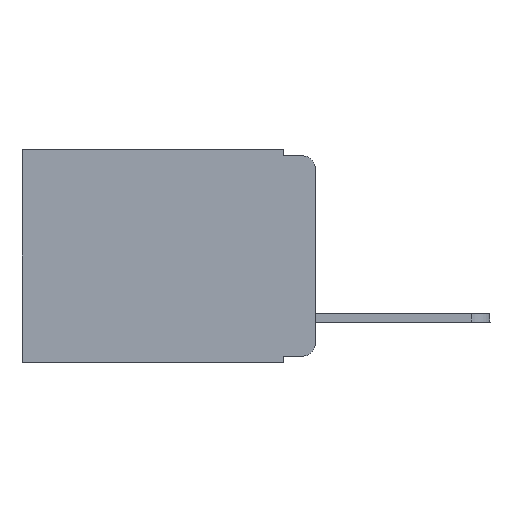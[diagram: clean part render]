
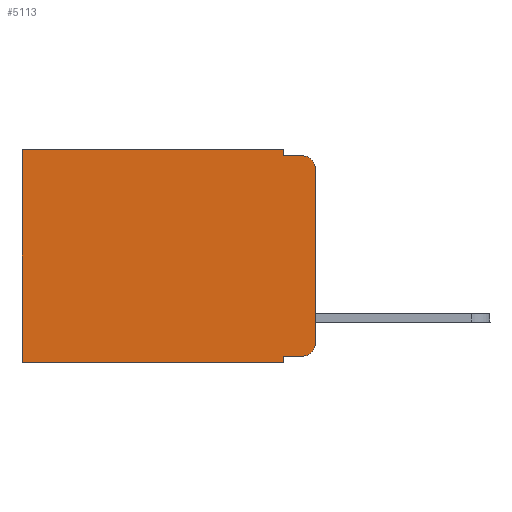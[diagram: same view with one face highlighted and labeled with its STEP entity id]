
A CAD part, left-side view. The second image highlights one B-rep face of the part: STEP entity #5113.
In plain terms, the highlighted planar face has unit normal (-1, 0, 0).
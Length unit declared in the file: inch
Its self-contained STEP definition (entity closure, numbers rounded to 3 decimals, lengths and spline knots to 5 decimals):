
#17 = DIRECTION ( 'NONE',  ( 0., 0., -1. ) ) ;
#591 = PLANE ( 'NONE',  #11629 ) ;
#739 = DIRECTION ( 'NONE',  ( 0., 0., -1. ) ) ;
#853 = LINE ( 'NONE', #16244, #5531 ) ;
#1234 = CARTESIAN_POINT ( 'NONE',  ( 0.298, 0.051, 0. ) ) ;
#1380 = VERTEX_POINT ( 'NONE', #17271 ) ;
#1464 = VERTEX_POINT ( 'NONE', #20986 ) ;
#1533 = DIRECTION ( 'NONE',  ( 0., 1., 0. ) ) ;
#2459 = DIRECTION ( 'NONE',  ( 0., 0., -1. ) ) ;
#2589 = CARTESIAN_POINT ( 'NONE',  ( 0.298, 0.473, 0. ) ) ;
#2749 = FACE_OUTER_BOUND ( 'NONE', #15265, .T. ) ;
#2856 = CARTESIAN_POINT ( 'NONE',  ( 0.298, 0., -0.343 ) ) ;
#3019 = CARTESIAN_POINT ( 'NONE',  ( 0.298, 0.02, -0.03 ) ) ;
#3084 = EDGE_CURVE ( 'NONE', #10100, #23614, #7540, .T. ) ;
#3555 = DIRECTION ( 'NONE',  ( 0., -1., 0. ) ) ;
#3571 = CIRCLE ( 'NONE', #18740, 0.02 ) ;
#3617 = VERTEX_POINT ( 'NONE', #1234 ) ;
#3624 = VECTOR ( 'NONE', #3555, 39.37008 ) ;
#3719 = CARTESIAN_POINT ( 'NONE',  ( 0.298, 0., 0. ) ) ;
#4767 = VERTEX_POINT ( 'NONE', #15419 ) ;
#4901 = DIRECTION ( 'NONE',  ( -1., 0., 0. ) ) ;
#5113 = ADVANCED_FACE ( 'NONE', ( #2749 ), #591, .F. ) ;
#5512 = EDGE_CURVE ( 'NONE', #9753, #4767, #10423, .T. ) ;
#5520 = ORIENTED_EDGE ( 'NONE', *, *, #6827, .T. ) ;
#5531 = VECTOR ( 'NONE', #19740, 39.37008 ) ;
#5766 = CARTESIAN_POINT ( 'NONE',  ( 0.298, 0.051, 0. ) ) ;
#5913 = VECTOR ( 'NONE', #22279, 39.37008 ) ;
#6529 = CARTESIAN_POINT ( 'NONE',  ( 0.298, 0.02, -0.01 ) ) ;
#6827 = EDGE_CURVE ( 'NONE', #11213, #1464, #19860, .T. ) ;
#7049 = VERTEX_POINT ( 'NONE', #6529 ) ;
#7318 = CARTESIAN_POINT ( 'NONE',  ( 0.298, 0.473, 0. ) ) ;
#7363 = CARTESIAN_POINT ( 'NONE',  ( 0.298, 0.051, -0.01 ) ) ;
#7469 = EDGE_CURVE ( 'NONE', #3617, #11213, #9447, .T. ) ;
#7478 = ORIENTED_EDGE ( 'NONE', *, *, #7469, .T. ) ;
#7540 = LINE ( 'NONE', #8030, #15030 ) ;
#8030 = CARTESIAN_POINT ( 'NONE',  ( 0.298, 0.051, -0.333 ) ) ;
#8277 = ORIENTED_EDGE ( 'NONE', *, *, #13677, .T. ) ;
#8878 = LINE ( 'NONE', #7363, #3624 ) ;
#8974 = VECTOR ( 'NONE', #18489, 39.37008 ) ;
#9447 = LINE ( 'NONE', #16238, #23856 ) ;
#9753 = VERTEX_POINT ( 'NONE', #10094 ) ;
#9776 = EDGE_CURVE ( 'NONE', #10100, #11954, #853, .T. ) ;
#10036 = DIRECTION ( 'NONE',  ( 1., 0., 0. ) ) ;
#10094 = CARTESIAN_POINT ( 'NONE',  ( 0.298, 0., -0.03 ) ) ;
#10100 = VERTEX_POINT ( 'NONE', #21640 ) ;
#10111 = DIRECTION ( 'NONE',  ( 0., 0., -1. ) ) ;
#10423 = LINE ( 'NONE', #3719, #8974 ) ;
#11213 = VERTEX_POINT ( 'NONE', #2589 ) ;
#11453 = LINE ( 'NONE', #5766, #5913 ) ;
#11629 = AXIS2_PLACEMENT_3D ( 'NONE', #21080, #10036, #739 ) ;
#11696 = EDGE_CURVE ( 'NONE', #1380, #7049, #8878, .T. ) ;
#11954 = VERTEX_POINT ( 'NONE', #16940 ) ;
#13580 = CARTESIAN_POINT ( 'NONE',  ( 0.298, 0.02, -0.333 ) ) ;
#13677 = EDGE_CURVE ( 'NONE', #9753, #7049, #22466, .T. ) ;
#14685 = ORIENTED_EDGE ( 'NONE', *, *, #16491, .T. ) ;
#15030 = VECTOR ( 'NONE', #22790, 39.37008 ) ;
#15265 = EDGE_LOOP ( 'NONE', ( #16723, #8277, #23164, #21544, #7478, #5520, #23516, #18592, #19074, #14685 ) ) ;
#15419 = CARTESIAN_POINT ( 'NONE',  ( 0.298, 0., -0.313 ) ) ;
#16238 = CARTESIAN_POINT ( 'NONE',  ( 0.298, 0., 0. ) ) ;
#16244 = CARTESIAN_POINT ( 'NONE',  ( 0.298, 0.051, 0. ) ) ;
#16491 = EDGE_CURVE ( 'NONE', #23614, #4767, #3571, .T. ) ;
#16723 = ORIENTED_EDGE ( 'NONE', *, *, #5512, .F. ) ;
#16940 = CARTESIAN_POINT ( 'NONE',  ( 0.298, 0.051, -0.343 ) ) ;
#17223 = DIRECTION ( 'NONE',  ( -1., 0., 0. ) ) ;
#17271 = CARTESIAN_POINT ( 'NONE',  ( 0.298, 0.051, -0.01 ) ) ;
#17485 = VECTOR ( 'NONE', #17, 39.37008 ) ;
#18489 = DIRECTION ( 'NONE',  ( 0., 0., -1. ) ) ;
#18592 = ORIENTED_EDGE ( 'NONE', *, *, #9776, .F. ) ;
#18740 = AXIS2_PLACEMENT_3D ( 'NONE', #20939, #17223, #2459 ) ;
#19074 = ORIENTED_EDGE ( 'NONE', *, *, #3084, .T. ) ;
#19235 = EDGE_CURVE ( 'NONE', #11954, #1464, #19611, .T. ) ;
#19611 = LINE ( 'NONE', #2856, #23378 ) ;
#19740 = DIRECTION ( 'NONE',  ( 0., 0., -1. ) ) ;
#19860 = LINE ( 'NONE', #7318, #17485 ) ;
#20939 = CARTESIAN_POINT ( 'NONE',  ( 0.298, 0.02, -0.313 ) ) ;
#20986 = CARTESIAN_POINT ( 'NONE',  ( 0.298, 0.473, -0.343 ) ) ;
#21080 = CARTESIAN_POINT ( 'NONE',  ( 0.298, 0., 0. ) ) ;
#21438 = EDGE_CURVE ( 'NONE', #3617, #1380, #11453, .T. ) ;
#21544 = ORIENTED_EDGE ( 'NONE', *, *, #21438, .F. ) ;
#21640 = CARTESIAN_POINT ( 'NONE',  ( 0.298, 0.051, -0.333 ) ) ;
#22132 = AXIS2_PLACEMENT_3D ( 'NONE', #3019, #4901, #10111 ) ;
#22279 = DIRECTION ( 'NONE',  ( 0., 0., -1. ) ) ;
#22466 = CIRCLE ( 'NONE', #22132, 0.02 ) ;
#22790 = DIRECTION ( 'NONE',  ( 0., -1., 0. ) ) ;
#22904 = DIRECTION ( 'NONE',  ( 0., 1., 0. ) ) ;
#23164 = ORIENTED_EDGE ( 'NONE', *, *, #11696, .F. ) ;
#23378 = VECTOR ( 'NONE', #22904, 39.37008 ) ;
#23516 = ORIENTED_EDGE ( 'NONE', *, *, #19235, .F. ) ;
#23614 = VERTEX_POINT ( 'NONE', #13580 ) ;
#23856 = VECTOR ( 'NONE', #1533, 39.37008 ) ;
